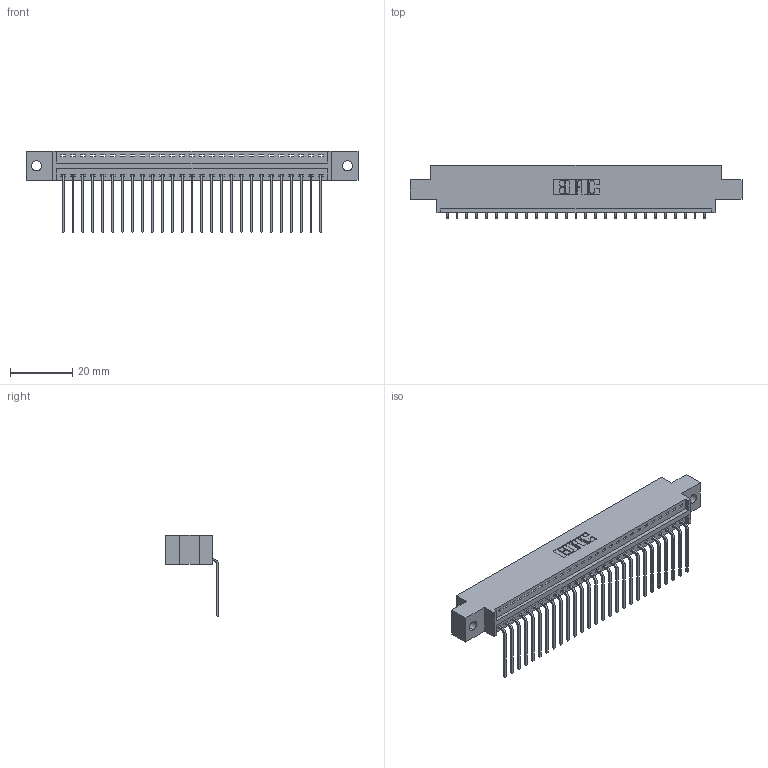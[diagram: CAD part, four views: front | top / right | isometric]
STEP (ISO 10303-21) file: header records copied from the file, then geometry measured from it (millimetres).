
FILE_DESCRIPTION (( 'STEP AP203' ), '1' );
FILE_NAME ('396-027-559-602.STEP', '2019-10-31T21:33:55', ( '' ), ( '' ), 'SwSTEP 2.0', 'SolidWorks 2016', '' );
FILE_SCHEMA (( 'CONFIG_CONTROL_DESIGN' ));
Length unit declared in the file: inch
Products named in the file (3): 346 Part_0.170 Offset - 0.128 Dia; 396-027-559-602; 345-292-001_558 559 Tail - 1
Assembly tree (28 placements, depth 2):
  396-027-559-602
    346 Part_0.170 Offset - 0.128 Dia
    345-292-001_558 559 Tail - 1  x27
Bounding box: 106.3 x 17.08 x 26.16 mm (x, y, z)
Volume: 9970.5 mm3; surface area: 12725.7 mm2
Topology: 28 solids, 28 shells, 1746 faces, 5255 edges, 3466 vertices
Faces by surface type: plane 1214, cylinder 532
Entity records: 18995 total; most frequent: CARTESIAN_POINT 3269, ORIENTED_EDGE 3230, DIRECTION 2901, EDGE_CURVE 1615, LINE 1375, VECTOR 1375, VERTEX_POINT 1074, AXIS2_PLACEMENT_3D 763
